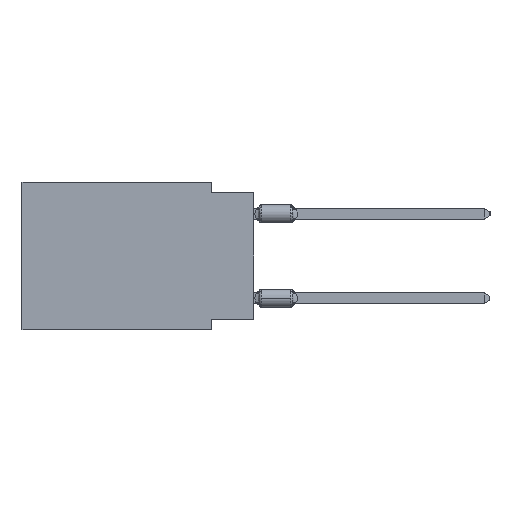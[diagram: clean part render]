
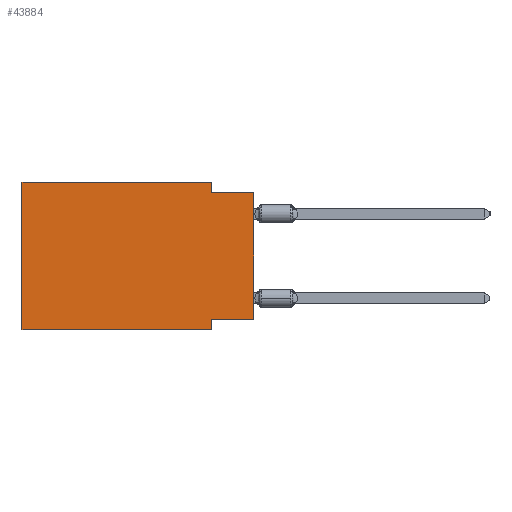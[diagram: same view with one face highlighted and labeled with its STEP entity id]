
A CAD part, left-side view. The second image highlights one B-rep face of the part: STEP entity #43884.
In plain terms, the highlighted planar face has unit normal (-1, 0, 0).
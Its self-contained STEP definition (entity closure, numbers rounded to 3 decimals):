
#9 = CARTESIAN_POINT ( 'NONE',  ( 0., 0., -0.635 ) ) ;
#195 = LINE ( 'NONE', #39441, #11034 ) ;
#797 = VECTOR ( 'NONE', #8554, 1000. ) ;
#1846 = AXIS2_PLACEMENT_3D ( 'NONE', #32875, #36420, #4023 ) ;
#1969 = EDGE_CURVE ( 'NONE', #24037, #32431, #44907, .T. ) ;
#2482 = EDGE_CURVE ( 'NONE', #24037, #32590, #11400, .T. ) ;
#3077 = VECTOR ( 'NONE', #17325, 1000. ) ;
#4023 = DIRECTION ( 'NONE',  ( 0., 0., -1. ) ) ;
#4514 = PLANE ( 'NONE',  #1846 ) ;
#4606 = CARTESIAN_POINT ( 'NONE',  ( 0., 13.97, 0. ) ) ;
#4944 = CARTESIAN_POINT ( 'NONE',  ( 0., 2.54, -8.89 ) ) ;
#5078 = CARTESIAN_POINT ( 'NONE',  ( 0., 2.54, -8.89 ) ) ;
#5263 = ORIENTED_EDGE ( 'NONE', *, *, #18369, .F. ) ;
#5628 = EDGE_CURVE ( 'NONE', #30460, #40124, #17779, .T. ) ;
#6892 = VECTOR ( 'NONE', #30125, 1000. ) ;
#7108 = ORIENTED_EDGE ( 'NONE', *, *, #1969, .F. ) ;
#8554 = DIRECTION ( 'NONE',  ( 0., -1., 0. ) ) ;
#9313 = VECTOR ( 'NONE', #26914, 1000. ) ;
#10806 = ORIENTED_EDGE ( 'NONE', *, *, #2482, .T. ) ;
#11034 = VECTOR ( 'NONE', #22185, 1000. ) ;
#11400 = LINE ( 'NONE', #43313, #16174 ) ;
#11455 = DIRECTION ( 'NONE',  ( 0., -1., 0. ) ) ;
#11629 = VERTEX_POINT ( 'NONE', #31995 ) ;
#11896 = CARTESIAN_POINT ( 'NONE',  ( 0., 2.54, -8.255 ) ) ;
#13386 = DIRECTION ( 'NONE',  ( 0., -1., 0. ) ) ;
#14168 = ORIENTED_EDGE ( 'NONE', *, *, #30255, .T. ) ;
#14881 = VERTEX_POINT ( 'NONE', #4944 ) ;
#15186 = CARTESIAN_POINT ( 'NONE',  ( 0., 0., -0.635 ) ) ;
#15654 = CARTESIAN_POINT ( 'NONE',  ( 0., 13.97, 0. ) ) ;
#16174 = VECTOR ( 'NONE', #29130, 1000. ) ;
#17325 = DIRECTION ( 'NONE',  ( 0., 0., 1. ) ) ;
#17779 = LINE ( 'NONE', #36216, #3077 ) ;
#17911 = EDGE_LOOP ( 'NONE', ( #10806, #37870, #5263, #22247, #30315, #14168, #34136, #7108 ) ) ;
#18369 = EDGE_CURVE ( 'NONE', #11629, #36916, #195, .T. ) ;
#19033 = LINE ( 'NONE', #5078, #6892 ) ;
#21758 = FACE_OUTER_BOUND ( 'NONE', #17911, .T. ) ;
#22185 = DIRECTION ( 'NONE',  ( 0., 0., -1. ) ) ;
#22247 = ORIENTED_EDGE ( 'NONE', *, *, #40720, .F. ) ;
#23959 = VECTOR ( 'NONE', #13386, 1000. ) ;
#24037 = VERTEX_POINT ( 'NONE', #28907 ) ;
#26914 = DIRECTION ( 'NONE',  ( 0., 1., 0. ) ) ;
#27564 = LINE ( 'NONE', #37755, #23959 ) ;
#27936 = EDGE_CURVE ( 'NONE', #36916, #32590, #29124, .T. ) ;
#28907 = CARTESIAN_POINT ( 'NONE',  ( 0., 0., -8.255 ) ) ;
#29124 = LINE ( 'NONE', #15186, #797 ) ;
#29130 = DIRECTION ( 'NONE',  ( 0., 0., 1. ) ) ;
#30125 = DIRECTION ( 'NONE',  ( 0., 0., -1. ) ) ;
#30255 = EDGE_CURVE ( 'NONE', #30460, #14881, #27564, .T. ) ;
#30315 = ORIENTED_EDGE ( 'NONE', *, *, #5628, .F. ) ;
#30460 = VERTEX_POINT ( 'NONE', #35821 ) ;
#31995 = CARTESIAN_POINT ( 'NONE',  ( 0., 2.54, 0. ) ) ;
#32431 = VERTEX_POINT ( 'NONE', #11896 ) ;
#32590 = VERTEX_POINT ( 'NONE', #9 ) ;
#32875 = CARTESIAN_POINT ( 'NONE',  ( 0., 13.97, 0. ) ) ;
#33675 = LINE ( 'NONE', #4606, #36334 ) ;
#34136 = ORIENTED_EDGE ( 'NONE', *, *, #40751, .F. ) ;
#35821 = CARTESIAN_POINT ( 'NONE',  ( 0., 13.97, -8.89 ) ) ;
#36216 = CARTESIAN_POINT ( 'NONE',  ( 0., 13.97, 0. ) ) ;
#36334 = VECTOR ( 'NONE', #11455, 1000. ) ;
#36420 = DIRECTION ( 'NONE',  ( 1., 0., 0. ) ) ;
#36916 = VERTEX_POINT ( 'NONE', #45850 ) ;
#37755 = CARTESIAN_POINT ( 'NONE',  ( 0., 13.97, -8.89 ) ) ;
#37870 = ORIENTED_EDGE ( 'NONE', *, *, #27936, .F. ) ;
#38263 = CARTESIAN_POINT ( 'NONE',  ( 0., 0., -8.255 ) ) ;
#39441 = CARTESIAN_POINT ( 'NONE',  ( 0., 2.54, 0. ) ) ;
#40124 = VERTEX_POINT ( 'NONE', #15654 ) ;
#40720 = EDGE_CURVE ( 'NONE', #40124, #11629, #33675, .T. ) ;
#40751 = EDGE_CURVE ( 'NONE', #32431, #14881, #19033, .T. ) ;
#43313 = CARTESIAN_POINT ( 'NONE',  ( 0., 0., 0. ) ) ;
#43884 = ADVANCED_FACE ( 'NONE', ( #21758 ), #4514, .F. ) ;
#44907 = LINE ( 'NONE', #38263, #9313 ) ;
#45850 = CARTESIAN_POINT ( 'NONE',  ( 0., 2.54, -0.635 ) ) ;
